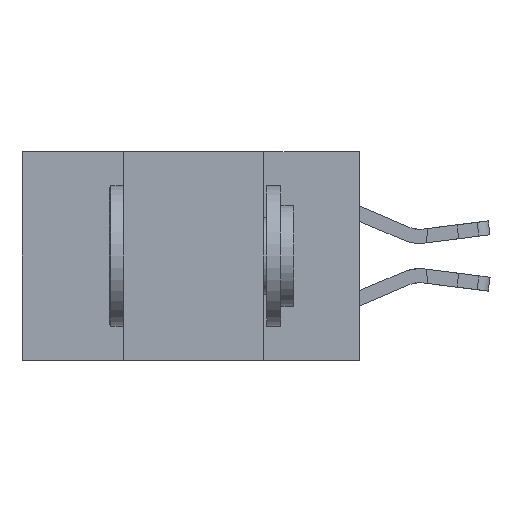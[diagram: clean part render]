
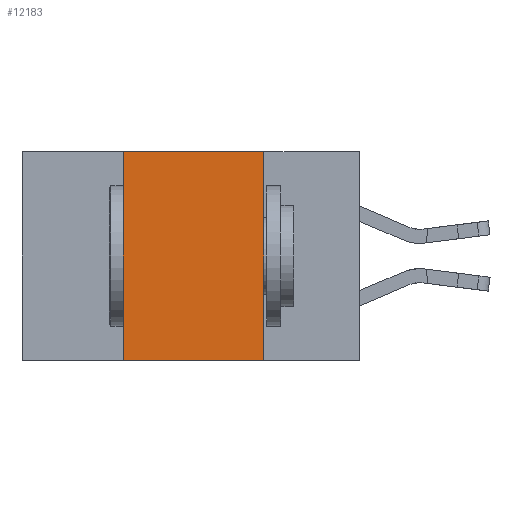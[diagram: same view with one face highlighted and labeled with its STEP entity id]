
A CAD part, left-side view. The second image highlights one B-rep face of the part: STEP entity #12183.
In plain terms, the highlighted planar face has unit normal (-1, 0, 0).
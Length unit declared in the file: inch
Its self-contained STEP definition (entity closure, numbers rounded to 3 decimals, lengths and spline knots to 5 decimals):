
#1708 = EDGE_LOOP ( 'NONE', ( #10945, #26943, #27479, #8562 ) ) ;
#3036 = CARTESIAN_POINT ( 'NONE',  ( 0., 0.42, 0. ) ) ;
#4746 = VERTEX_POINT ( 'NONE', #31594 ) ;
#5846 = VERTEX_POINT ( 'NONE', #27758 ) ;
#6519 = VECTOR ( 'NONE', #28418, 39.37008 ) ;
#7740 = DIRECTION ( 'NONE',  ( 1., 0., 0. ) ) ;
#8562 = ORIENTED_EDGE ( 'NONE', *, *, #19141, .T. ) ;
#8662 = FACE_OUTER_BOUND ( 'NONE', #1708, .T. ) ;
#10159 = VECTOR ( 'NONE', #13136, 39.37008 ) ;
#10812 = EDGE_CURVE ( 'NONE', #4746, #5846, #30160, .T. ) ;
#10945 = ORIENTED_EDGE ( 'NONE', *, *, #29564, .F. ) ;
#12127 = LINE ( 'NONE', #19536, #32323 ) ;
#12183 = ADVANCED_FACE ( 'NONE', ( #8662 ), #25111, .F. ) ;
#12764 = VECTOR ( 'NONE', #13188, 39.37008 ) ;
#12937 = LINE ( 'NONE', #24111, #10159 ) ;
#13136 = DIRECTION ( 'NONE',  ( 0., -1., 0. ) ) ;
#13188 = DIRECTION ( 'NONE',  ( 0., 0., 1. ) ) ;
#14077 = VERTEX_POINT ( 'NONE', #24268 ) ;
#19141 = EDGE_CURVE ( 'NONE', #4746, #14077, #12937, .T. ) ;
#19536 = CARTESIAN_POINT ( 'NONE',  ( 0., 0.6, 0. ) ) ;
#19896 = EDGE_CURVE ( 'NONE', #5846, #33350, #12127, .T. ) ;
#20566 = CARTESIAN_POINT ( 'NONE',  ( 0., 0.6, 0. ) ) ;
#21832 = LINE ( 'NONE', #25689, #6519 ) ;
#24111 = CARTESIAN_POINT ( 'NONE',  ( 0., 0.6, -0.37 ) ) ;
#24268 = CARTESIAN_POINT ( 'NONE',  ( 0., 0.17, -0.37 ) ) ;
#25111 = PLANE ( 'NONE',  #28006 ) ;
#25689 = CARTESIAN_POINT ( 'NONE',  ( 0., 0.17, 0. ) ) ;
#26943 = ORIENTED_EDGE ( 'NONE', *, *, #19896, .F. ) ;
#27133 = DIRECTION ( 'NONE',  ( 0., -1., 0. ) ) ;
#27479 = ORIENTED_EDGE ( 'NONE', *, *, #10812, .F. ) ;
#27758 = CARTESIAN_POINT ( 'NONE',  ( 0., 0.42, 0. ) ) ;
#27842 = DIRECTION ( 'NONE',  ( 0., 0., -1. ) ) ;
#27887 = CARTESIAN_POINT ( 'NONE',  ( 0., 0.17, 0. ) ) ;
#28006 = AXIS2_PLACEMENT_3D ( 'NONE', #20566, #7740, #27842 ) ;
#28418 = DIRECTION ( 'NONE',  ( 0., 0., -1. ) ) ;
#29564 = EDGE_CURVE ( 'NONE', #33350, #14077, #21832, .T. ) ;
#30160 = LINE ( 'NONE', #3036, #12764 ) ;
#31594 = CARTESIAN_POINT ( 'NONE',  ( 0., 0.42, -0.37 ) ) ;
#32323 = VECTOR ( 'NONE', #27133, 39.37008 ) ;
#33350 = VERTEX_POINT ( 'NONE', #27887 ) ;
